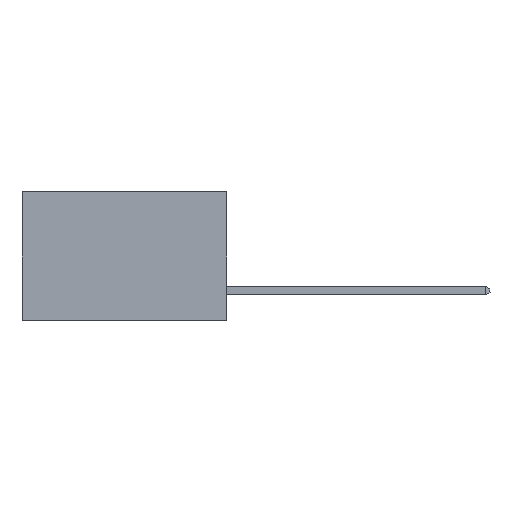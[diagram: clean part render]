
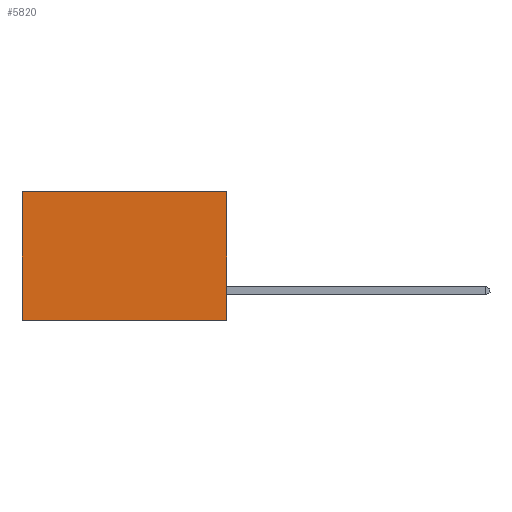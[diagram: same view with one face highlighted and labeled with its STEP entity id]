
A CAD part, left-side view. The second image highlights one B-rep face of the part: STEP entity #5820.
In plain terms, the highlighted planar face has unit normal (-1, 0, 0).
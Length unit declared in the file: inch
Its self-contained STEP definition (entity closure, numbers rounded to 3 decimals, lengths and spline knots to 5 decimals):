
#772 = AXIS2_PLACEMENT_3D ( 'NONE', #5127, #5114, #5097 ) ;
#990 = ORIENTED_EDGE ( 'NONE', *, *, #9263, .T. ) ;
#1017 = ORIENTED_EDGE ( 'NONE', *, *, #3202, .F. ) ;
#1062 = ORIENTED_EDGE ( 'NONE', *, *, #8589, .F. ) ;
#1073 = ORIENTED_EDGE ( 'NONE', *, *, #5602, .T. ) ;
#1458 = CARTESIAN_POINT ( 'NONE',  ( 0.277, 0.59, 0. ) ) ;
#2088 = VERTEX_POINT ( 'NONE', #6555 ) ;
#2210 = LINE ( 'NONE', #10424, #10587 ) ;
#2234 = VERTEX_POINT ( 'NONE', #8089 ) ;
#2257 = CARTESIAN_POINT ( 'NONE',  ( 0.277, 0.59, -0.37 ) ) ;
#2426 = VECTOR ( 'NONE', #5534, 39.37008 ) ;
#3202 = EDGE_CURVE ( 'NONE', #10194, #2088, #2210, .T. ) ;
#3235 = VERTEX_POINT ( 'NONE', #1458 ) ;
#4501 = LINE ( 'NONE', #6469, #8629 ) ;
#5061 = DIRECTION ( 'NONE',  ( 0., 1., 0. ) ) ;
#5097 = DIRECTION ( 'NONE',  ( 0., 0., -1. ) ) ;
#5114 = DIRECTION ( 'NONE',  ( 1., 0., 0. ) ) ;
#5127 = CARTESIAN_POINT ( 'NONE',  ( 0.277, 0., -0.37 ) ) ;
#5156 = PLANE ( 'NONE',  #772 ) ;
#5534 = DIRECTION ( 'NONE',  ( 0., 0., -1. ) ) ;
#5602 = EDGE_CURVE ( 'NONE', #2234, #3235, #6400, .T. ) ;
#5820 = ADVANCED_FACE ( 'NONE', ( #6531 ), #5156, .F. ) ;
#6400 = LINE ( 'NONE', #8341, #8357 ) ;
#6469 = CARTESIAN_POINT ( 'NONE',  ( 0.277, 0., -0.37 ) ) ;
#6531 = FACE_OUTER_BOUND ( 'NONE', #9231, .T. ) ;
#6555 = CARTESIAN_POINT ( 'NONE',  ( 0.277, 0.59, -0.37 ) ) ;
#6789 = LINE ( 'NONE', #2257, #2426 ) ;
#7512 = CARTESIAN_POINT ( 'NONE',  ( 0.277, 0., -0.37 ) ) ;
#8089 = CARTESIAN_POINT ( 'NONE',  ( 0.277, 0., 0. ) ) ;
#8148 = DIRECTION ( 'NONE',  ( 0., 0., -1. ) ) ;
#8179 = DIRECTION ( 'NONE',  ( 0., 1., 0. ) ) ;
#8341 = CARTESIAN_POINT ( 'NONE',  ( 0.277, 0., 0. ) ) ;
#8357 = VECTOR ( 'NONE', #8179, 39.37008 ) ;
#8589 = EDGE_CURVE ( 'NONE', #2234, #10194, #4501, .T. ) ;
#8629 = VECTOR ( 'NONE', #8148, 39.37008 ) ;
#9231 = EDGE_LOOP ( 'NONE', ( #990, #1017, #1062, #1073 ) ) ;
#9263 = EDGE_CURVE ( 'NONE', #3235, #2088, #6789, .T. ) ;
#10194 = VERTEX_POINT ( 'NONE', #7512 ) ;
#10424 = CARTESIAN_POINT ( 'NONE',  ( 0.277, 0., -0.37 ) ) ;
#10587 = VECTOR ( 'NONE', #5061, 39.37008 ) ;
